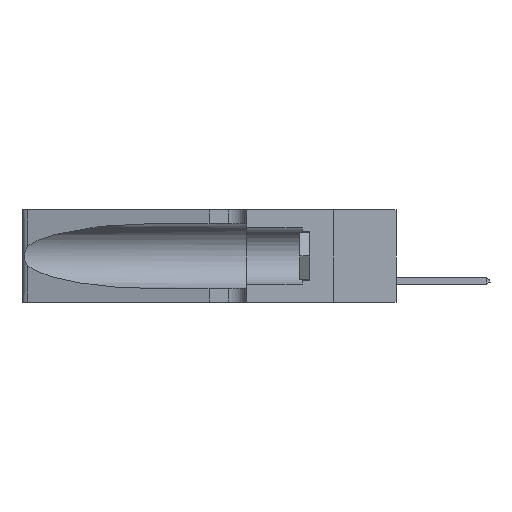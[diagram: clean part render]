
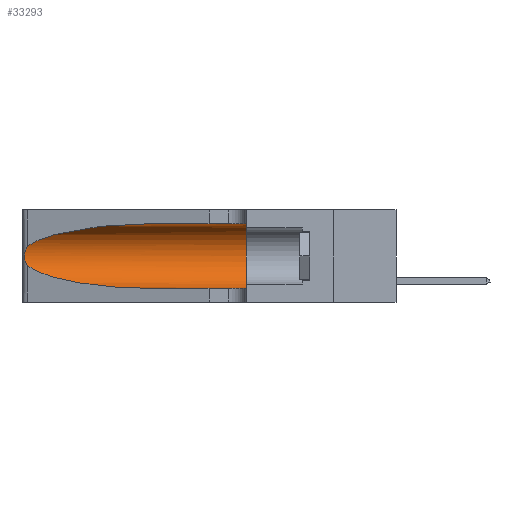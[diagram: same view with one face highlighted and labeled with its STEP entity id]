
A CAD part, left-side view. The second image highlights one B-rep face of the part: STEP entity #33293.
In plain terms, the highlighted cylindrical face has radius 3.308 mm (diameter 6.617 mm), a partial arc.
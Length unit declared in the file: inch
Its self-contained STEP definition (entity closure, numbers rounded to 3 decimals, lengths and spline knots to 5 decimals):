
#28 = VERTEX_POINT ( 'NONE', #15582 ) ;
#343 = DIRECTION ( 'NONE',  ( 0., 0., -1. ) ) ;
#1422 = CARTESIAN_POINT ( 'NONE',  ( 0.1305, 1.61858, 0.05475 ) ) ;
#2689 = CARTESIAN_POINT ( 'NONE',  ( 0.1305, 0.35, 0.31525 ) ) ;
#3485 = CARTESIAN_POINT ( 'NONE',  ( 0.1305, 0.72297, 0.31525 ) ) ;
#5185 = CARTESIAN_POINT ( 'NONE',  ( 0.25487, 1.22718, 0.22369 ) ) ;
#6593 = CARTESIAN_POINT ( 'NONE',  ( 0.18966, 0.96281, 0.31525 ) ) ;
#7071 = VERTEX_POINT ( 'NONE', #27607 ) ;
#7581 = DIRECTION ( 'NONE',  ( 0., -1., 0. ) ) ;
#7775 = CARTESIAN_POINT ( 'NONE',  ( 0.1305, 0.35, 0.05475 ) ) ;
#7947 =( BOUNDED_CURVE ( )  B_SPLINE_CURVE ( 3, ( #30602, #25721, #29565, #8521 ),
 .UNSPECIFIED., .F., .T. ) 
 B_SPLINE_CURVE_WITH_KNOTS ( ( 4, 4 ),
 ( 3.44316, 4.71239 ),
 .UNSPECIFIED. ) 
 CURVE ( )  GEOMETRIC_REPRESENTATION_ITEM ( )  RATIONAL_B_SPLINE_CURVE ( ( 1., 0.87, 0.87, 1. ) ) 
 REPRESENTATION_ITEM ( '' )  );
#8115 = VERTEX_POINT ( 'NONE', #2689 ) ;
#8259 = FACE_OUTER_BOUND ( 'NONE', #20719, .T. ) ;
#8484 = EDGE_CURVE ( 'NONE', #35878, #28, #7947, .T. ) ;
#8521 = CARTESIAN_POINT ( 'NONE',  ( 0.1305, 0.72297, 0.05475 ) ) ;
#9141 = VERTEX_POINT ( 'NONE', #3485 ) ;
#12022 = DIRECTION ( 'NONE',  ( 0., -1., 0. ) ) ;
#12768 = EDGE_CURVE ( 'NONE', #9141, #7071, #25688, .T. ) ;
#13195 = CARTESIAN_POINT ( 'NONE',  ( 0.25639, 1.23186, 0.15144 ) ) ;
#13785 = AXIS2_PLACEMENT_3D ( 'NONE', #32269, #25177, #15208 ) ;
#14495 = CARTESIAN_POINT ( 'NONE',  ( 0.1305, 1.61858, 0.185 ) ) ;
#14631 = ORIENTED_EDGE ( 'NONE', *, *, #24162, .T. ) ;
#15087 = LINE ( 'NONE', #27891, #42039 ) ;
#15208 = DIRECTION ( 'NONE',  ( 0., 0., 1. ) ) ;
#15582 = CARTESIAN_POINT ( 'NONE',  ( 0.1305, 0.72297, 0.05475 ) ) ;
#16101 = CARTESIAN_POINT ( 'NONE',  ( 0.26075, 1.23896, 0.178 ) ) ;
#16579 = CARTESIAN_POINT ( 'NONE',  ( 0.25856, 1.23593, 0.16098 ) ) ;
#17678 = VERTEX_POINT ( 'NONE', #7775 ) ;
#17710 = EDGE_CURVE ( 'NONE', #9141, #8115, #15087, .T. ) ;
#18583 = CIRCLE ( 'NONE', #13785, 0.13025 ) ;
#19539 = B_SPLINE_CURVE_WITH_KNOTS ( 'NONE', 3,
 ( #5185, #33958, #19630, #23635, #30214, #37627, #23331, #16101, #41310, #16579, #40679, #13195, #44371, #44222 ),
 .UNSPECIFIED., .F., .F.,
 ( 4, 2, 2, 2, 2, 2, 4 ),
 ( 0., 0.00027, 0.00053, 0.00107, 0.0016, 0.00187, 0.00214 ),
 .UNSPECIFIED. ) ;
#19630 = CARTESIAN_POINT ( 'NONE',  ( 0.25639, 1.23184, 0.21858 ) ) ;
#20719 = EDGE_LOOP ( 'NONE', ( #39538, #38973, #24408, #14631, #21606, #34835 ) ) ;
#21606 = ORIENTED_EDGE ( 'NONE', *, *, #21957, .F. ) ;
#21957 = EDGE_CURVE ( 'NONE', #8115, #17678, #18583, .T. ) ;
#23331 = CARTESIAN_POINT ( 'NONE',  ( 0.26075, 1.23896, 0.19203 ) ) ;
#23635 = CARTESIAN_POINT ( 'NONE',  ( 0.25787, 1.23484, 0.2124 ) ) ;
#24162 = EDGE_CURVE ( 'NONE', #28, #17678, #24723, .T. ) ;
#24408 = ORIENTED_EDGE ( 'NONE', *, *, #8484, .T. ) ;
#24723 = LINE ( 'NONE', #1422, #35213 ) ;
#25177 = DIRECTION ( 'NONE',  ( 0., 1., 0. ) ) ;
#25688 =( BOUNDED_CURVE ( )  B_SPLINE_CURVE ( 3, ( #41615, #6593, #28353, #34135 ),
 .UNSPECIFIED., .F., .F. ) 
 B_SPLINE_CURVE_WITH_KNOTS ( ( 4, 4 ),
 ( 1.5708, 2.84003 ),
 .UNSPECIFIED. ) 
 CURVE ( )  GEOMETRIC_REPRESENTATION_ITEM ( )  RATIONAL_B_SPLINE_CURVE ( ( 1., 0.87, 0.87, 1. ) ) 
 REPRESENTATION_ITEM ( '' )  );
#25721 = CARTESIAN_POINT ( 'NONE',  ( 0.2373, 1.15595, 0.08982 ) ) ;
#27607 = CARTESIAN_POINT ( 'NONE',  ( 0.25487, 1.22718, 0.22369 ) ) ;
#27891 = CARTESIAN_POINT ( 'NONE',  ( 0.1305, 1.61858, 0.31525 ) ) ;
#28353 = CARTESIAN_POINT ( 'NONE',  ( 0.2373, 1.15595, 0.28018 ) ) ;
#29565 = CARTESIAN_POINT ( 'NONE',  ( 0.18966, 0.96281, 0.05475 ) ) ;
#30214 = CARTESIAN_POINT ( 'NONE',  ( 0.25854, 1.2359, 0.20912 ) ) ;
#30602 = CARTESIAN_POINT ( 'NONE',  ( 0.25487, 1.22718, 0.14631 ) ) ;
#30923 = EDGE_CURVE ( 'NONE', #7071, #35878, #19539, .T. ) ;
#31727 = AXIS2_PLACEMENT_3D ( 'NONE', #14495, #7581, #343 ) ;
#32269 = CARTESIAN_POINT ( 'NONE',  ( 0.1305, 0.35, 0.185 ) ) ;
#33293 = ADVANCED_FACE ( 'NONE', ( #8259 ), #42329, .F. ) ;
#33958 = CARTESIAN_POINT ( 'NONE',  ( 0.25555, 1.22994, 0.2215 ) ) ;
#34135 = CARTESIAN_POINT ( 'NONE',  ( 0.25487, 1.22718, 0.22369 ) ) ;
#34835 = ORIENTED_EDGE ( 'NONE', *, *, #17710, .F. ) ;
#35213 = VECTOR ( 'NONE', #42230, 39.37008 ) ;
#35878 = VERTEX_POINT ( 'NONE', #42982 ) ;
#37627 = CARTESIAN_POINT ( 'NONE',  ( 0.26018, 1.23835, 0.19895 ) ) ;
#38973 = ORIENTED_EDGE ( 'NONE', *, *, #30923, .T. ) ;
#39538 = ORIENTED_EDGE ( 'NONE', *, *, #12768, .T. ) ;
#40679 = CARTESIAN_POINT ( 'NONE',  ( 0.25789, 1.23486, 0.15765 ) ) ;
#41310 = CARTESIAN_POINT ( 'NONE',  ( 0.26017, 1.23833, 0.17102 ) ) ;
#41615 = CARTESIAN_POINT ( 'NONE',  ( 0.1305, 0.72297, 0.31525 ) ) ;
#42039 = VECTOR ( 'NONE', #12022, 39.37008 ) ;
#42230 = DIRECTION ( 'NONE',  ( 0., -1., 0. ) ) ;
#42329 = CYLINDRICAL_SURFACE ( 'NONE', #31727, 0.13025 ) ;
#42982 = CARTESIAN_POINT ( 'NONE',  ( 0.25487, 1.22718, 0.14631 ) ) ;
#44222 = CARTESIAN_POINT ( 'NONE',  ( 0.25487, 1.22718, 0.14631 ) ) ;
#44371 = CARTESIAN_POINT ( 'NONE',  ( 0.25555, 1.22993, 0.14849 ) ) ;
